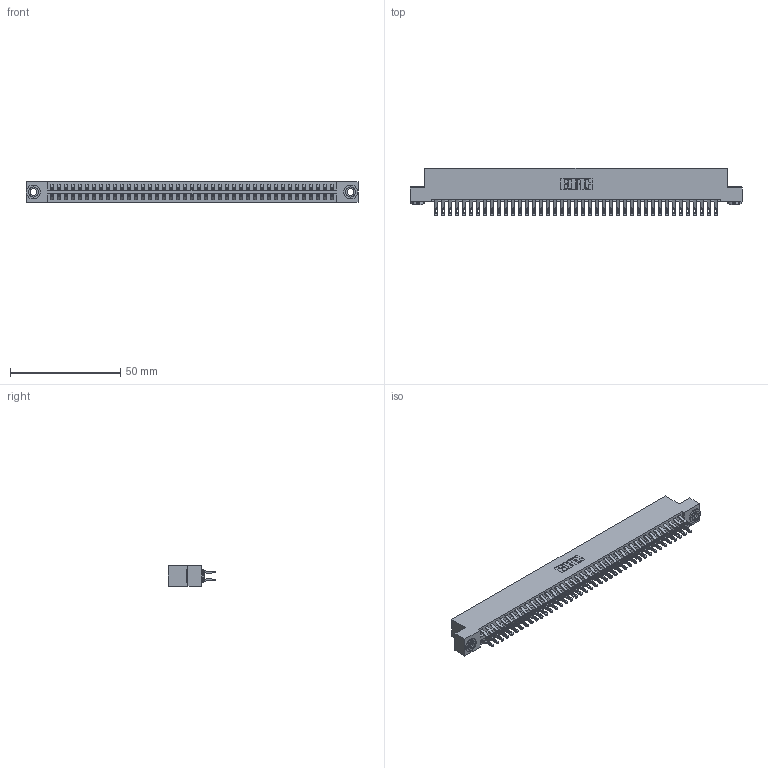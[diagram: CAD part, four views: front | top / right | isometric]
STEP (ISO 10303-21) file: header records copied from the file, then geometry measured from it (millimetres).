
FILE_DESCRIPTION (( 'STEP AP203' ), '1' );
FILE_NAME ('346-082-555-203.STEP', '2022-05-25T18:10:50', ( '' ), ( '' ), 'SwSTEP 2.0', 'SolidWorks 2020', '' );
FILE_SCHEMA (( 'CONFIG_CONTROL_DESIGN' ));
Length unit declared in the file: inch
Products named in the file (4): 346-082-555-203; 345-292-001_555 Tail; 345-250-002_345-250-002-102; 346 Part_Flush Mounting Lugs - 0.156 Dia-TH
Assembly tree (85 placements, depth 2):
  346-082-555-203
    346 Part_Flush Mounting Lugs - 0.156 Dia-TH
    345-292-001_555 Tail  x82
    345-250-002_345-250-002-102  x2
Bounding box: 150.75 x 21.46 x 9.4 mm (x, y, z)
Volume: 14931.3 mm3; surface area: 21604.9 mm2
Topology: 85 solids, 85 shells, 4930 faces, 15447 edges, 10294 vertices
Faces by surface type: plane 2806, cylinder 2116, cone 8
Entity records: 28284 total; most frequent: CARTESIAN_POINT 4679, ORIENTED_EDGE 4574, DIRECTION 4173, EDGE_CURVE 2287, LINE 1947, VECTOR 1947, VERTEX_POINT 1522, AXIS2_PLACEMENT_3D 1113
